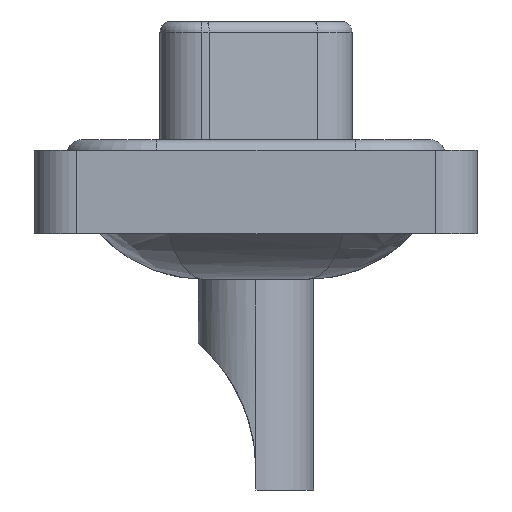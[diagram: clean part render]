
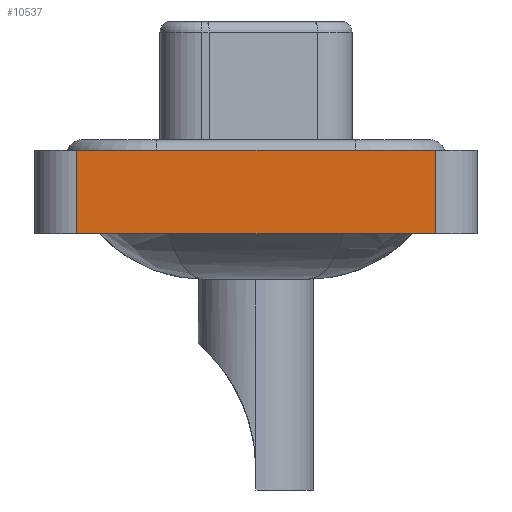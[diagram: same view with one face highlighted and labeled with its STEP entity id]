
A CAD part, left-side view. The second image highlights one B-rep face of the part: STEP entity #10537.
In plain terms, the highlighted planar face has unit normal (-1, 0, 0).
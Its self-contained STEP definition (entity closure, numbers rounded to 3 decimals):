
#841 = EDGE_CURVE ( 'NONE', #18285, #9023, #9951, .T. ) ;
#971 = CARTESIAN_POINT ( 'NONE',  ( -7.35, 8.55, -3.6 ) ) ;
#1451 = CARTESIAN_POINT ( 'NONE',  ( -7.35, -8.55, 0.4 ) ) ;
#2585 = LINE ( 'NONE', #9853, #8285 ) ;
#3176 = DIRECTION ( 'NONE',  ( 0., 0., 1. ) ) ;
#5191 = PLANE ( 'NONE',  #15858 ) ;
#5204 = EDGE_LOOP ( 'NONE', ( #14690, #23243, #12939, #5830 ) ) ;
#5830 = ORIENTED_EDGE ( 'NONE', *, *, #841, .T. ) ;
#6236 = EDGE_CURVE ( 'NONE', #18285, #8943, #10483, .T. ) ;
#6372 = DIRECTION ( 'NONE',  ( 0., -1., 0. ) ) ;
#7028 = VECTOR ( 'NONE', #19810, 1000. ) ;
#8285 = VECTOR ( 'NONE', #3176, 1000. ) ;
#8530 = DIRECTION ( 'NONE',  ( 0., 0., 1. ) ) ;
#8943 = VERTEX_POINT ( 'NONE', #14575 ) ;
#9023 = VERTEX_POINT ( 'NONE', #9677 ) ;
#9677 = CARTESIAN_POINT ( 'NONE',  ( -7.35, -8.55, -3.6 ) ) ;
#9853 = CARTESIAN_POINT ( 'NONE',  ( -7.35, -8.55, -3.6 ) ) ;
#9951 = LINE ( 'NONE', #11619, #18241 ) ;
#10483 = LINE ( 'NONE', #18019, #7028 ) ;
#10537 = ADVANCED_FACE ( 'NONE', ( #23202 ), #5191, .T. ) ;
#11619 = CARTESIAN_POINT ( 'NONE',  ( -7.35, -8.55, -3.6 ) ) ;
#11777 = EDGE_CURVE ( 'NONE', #9023, #18236, #2585, .T. ) ;
#12939 = ORIENTED_EDGE ( 'NONE', *, *, #6236, .F. ) ;
#14139 = CARTESIAN_POINT ( 'NONE',  ( -7.35, -8.55, -3.6 ) ) ;
#14575 = CARTESIAN_POINT ( 'NONE',  ( -7.35, 8.55, 0.4 ) ) ;
#14690 = ORIENTED_EDGE ( 'NONE', *, *, #11777, .T. ) ;
#15647 = CARTESIAN_POINT ( 'NONE',  ( -7.35, -8.55, 0.4 ) ) ;
#15858 = AXIS2_PLACEMENT_3D ( 'NONE', #14139, #19391, #8530 ) ;
#16295 = VECTOR ( 'NONE', #23393, 1000. ) ;
#18019 = CARTESIAN_POINT ( 'NONE',  ( -7.35, 8.55, -3.6 ) ) ;
#18153 = LINE ( 'NONE', #1451, #16295 ) ;
#18236 = VERTEX_POINT ( 'NONE', #15647 ) ;
#18241 = VECTOR ( 'NONE', #6372, 1000. ) ;
#18285 = VERTEX_POINT ( 'NONE', #971 ) ;
#18374 = EDGE_CURVE ( 'NONE', #8943, #18236, #18153, .T. ) ;
#19391 = DIRECTION ( 'NONE',  ( -1., 0., 0. ) ) ;
#19810 = DIRECTION ( 'NONE',  ( 0., 0., 1. ) ) ;
#23202 = FACE_OUTER_BOUND ( 'NONE', #5204, .T. ) ;
#23243 = ORIENTED_EDGE ( 'NONE', *, *, #18374, .F. ) ;
#23393 = DIRECTION ( 'NONE',  ( 0., -1., 0. ) ) ;
